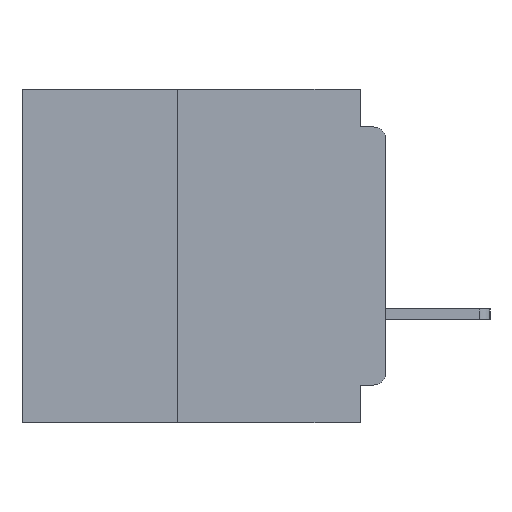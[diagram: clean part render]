
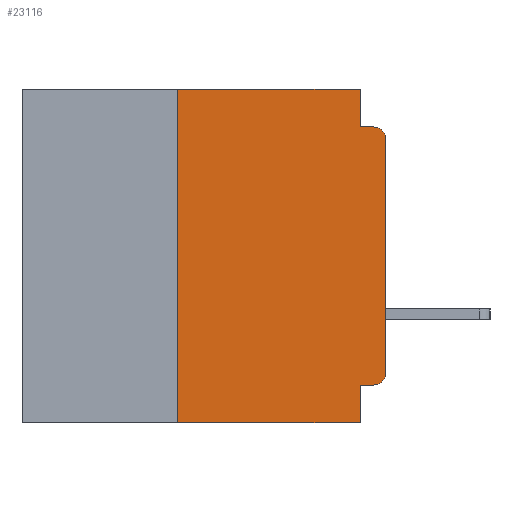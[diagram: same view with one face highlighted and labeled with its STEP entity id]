
A CAD part, left-side view. The second image highlights one B-rep face of the part: STEP entity #23116.
In plain terms, the highlighted planar face has unit normal (-1, 0, 0).
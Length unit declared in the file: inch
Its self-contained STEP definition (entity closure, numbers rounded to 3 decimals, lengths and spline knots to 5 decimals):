
#888 = EDGE_CURVE ( 'NONE', #4619, #17819, #34045, .T. ) ;
#2094 = CIRCLE ( 'NONE', #13594, 0.015 ) ;
#2115 = CARTESIAN_POINT ( 'NONE',  ( 0., 0.031, -0.4 ) ) ;
#2514 = CARTESIAN_POINT ( 'NONE',  ( 0., 0.031, -0.355 ) ) ;
#3103 = EDGE_CURVE ( 'NONE', #8477, #9097, #13351, .T. ) ;
#3969 = LINE ( 'NONE', #42979, #28569 ) ;
#4619 = VERTEX_POINT ( 'NONE', #24319 ) ;
#5118 = CARTESIAN_POINT ( 'NONE',  ( 0., 0.031, 0. ) ) ;
#5341 = DIRECTION ( 'NONE',  ( 0., 0., 1. ) ) ;
#5446 = EDGE_CURVE ( 'NONE', #5993, #7197, #28767, .T. ) ;
#5721 = VECTOR ( 'NONE', #15333, 39.37008 ) ;
#5993 = VERTEX_POINT ( 'NONE', #18700 ) ;
#6261 = CARTESIAN_POINT ( 'NONE',  ( 0., 0.031, -0.045 ) ) ;
#6871 = VECTOR ( 'NONE', #11600, 39.37008 ) ;
#7197 = VERTEX_POINT ( 'NONE', #2514 ) ;
#7807 = AXIS2_PLACEMENT_3D ( 'NONE', #40849, #14601, #37731 ) ;
#7888 = AXIS2_PLACEMENT_3D ( 'NONE', #30933, #22339, #20703 ) ;
#8477 = VERTEX_POINT ( 'NONE', #26603 ) ;
#8787 = ORIENTED_EDGE ( 'NONE', *, *, #8852, .F. ) ;
#8852 = EDGE_CURVE ( 'NONE', #7197, #25153, #23543, .T. ) ;
#8934 = CARTESIAN_POINT ( 'NONE',  ( 0., 0.031, -0.4 ) ) ;
#9097 = VERTEX_POINT ( 'NONE', #16725 ) ;
#10554 = ORIENTED_EDGE ( 'NONE', *, *, #17882, .F. ) ;
#10706 = CARTESIAN_POINT ( 'NONE',  ( 0., 0.015, -0.34 ) ) ;
#11222 = PLANE ( 'NONE',  #7807 ) ;
#11600 = DIRECTION ( 'NONE',  ( 0., -1., 0. ) ) ;
#11652 = EDGE_LOOP ( 'NONE', ( #22100, #34295, #29966, #24642, #14108, #10554, #26506, #8787, #36205, #35474 ) ) ;
#11753 = CARTESIAN_POINT ( 'NONE',  ( 0., 0.015, -0.045 ) ) ;
#12036 = CARTESIAN_POINT ( 'NONE',  ( 0., 0.25, -0.4 ) ) ;
#13015 = VERTEX_POINT ( 'NONE', #6261 ) ;
#13351 = LINE ( 'NONE', #34385, #38707 ) ;
#13594 = AXIS2_PLACEMENT_3D ( 'NONE', #10706, #33955, #14080 ) ;
#14080 = DIRECTION ( 'NONE',  ( 0., 0., -1. ) ) ;
#14108 = ORIENTED_EDGE ( 'NONE', *, *, #3103, .F. ) ;
#14601 = DIRECTION ( 'NONE',  ( 1., 0., 0. ) ) ;
#14740 = LINE ( 'NONE', #5118, #5721 ) ;
#15333 = DIRECTION ( 'NONE',  ( 0., 0., -1. ) ) ;
#15645 = EDGE_CURVE ( 'NONE', #39787, #25153, #3969, .T. ) ;
#15729 = VECTOR ( 'NONE', #28876, 39.37008 ) ;
#16725 = CARTESIAN_POINT ( 'NONE',  ( 0., 0.031, 0. ) ) ;
#17139 = DIRECTION ( 'NONE',  ( 0., 0., 1. ) ) ;
#17592 = FACE_OUTER_BOUND ( 'NONE', #11652, .T. ) ;
#17819 = VERTEX_POINT ( 'NONE', #11753 ) ;
#17882 = EDGE_CURVE ( 'NONE', #39787, #8477, #35673, .T. ) ;
#18700 = CARTESIAN_POINT ( 'NONE',  ( 0., 0.015, -0.355 ) ) ;
#20130 = EDGE_CURVE ( 'NONE', #9097, #13015, #14740, .T. ) ;
#20703 = DIRECTION ( 'NONE',  ( 0., 0., -1. ) ) ;
#22100 = ORIENTED_EDGE ( 'NONE', *, *, #41073, .T. ) ;
#22215 = CARTESIAN_POINT ( 'NONE',  ( 0., 0.25, -0.4 ) ) ;
#22339 = DIRECTION ( 'NONE',  ( -1., 0., 0. ) ) ;
#22647 = DIRECTION ( 'NONE',  ( 0., 1., 0. ) ) ;
#23116 = ADVANCED_FACE ( 'NONE', ( #17592 ), #11222, .F. ) ;
#23303 = DIRECTION ( 'NONE',  ( 0., -1., 0. ) ) ;
#23543 = LINE ( 'NONE', #8934, #15729 ) ;
#24319 = CARTESIAN_POINT ( 'NONE',  ( 0., 0., -0.06 ) ) ;
#24642 = ORIENTED_EDGE ( 'NONE', *, *, #20130, .F. ) ;
#25153 = VERTEX_POINT ( 'NONE', #2115 ) ;
#25642 = EDGE_CURVE ( 'NONE', #13015, #17819, #42145, .T. ) ;
#26506 = ORIENTED_EDGE ( 'NONE', *, *, #15645, .T. ) ;
#26603 = CARTESIAN_POINT ( 'NONE',  ( 0., 0.25, 0. ) ) ;
#26873 = VECTOR ( 'NONE', #5341, 39.37008 ) ;
#27188 = VERTEX_POINT ( 'NONE', #35729 ) ;
#28569 = VECTOR ( 'NONE', #23303, 39.37008 ) ;
#28767 = LINE ( 'NONE', #29280, #36529 ) ;
#28876 = DIRECTION ( 'NONE',  ( 0., 0., -1. ) ) ;
#29280 = CARTESIAN_POINT ( 'NONE',  ( 0., 0., -0.355 ) ) ;
#29966 = ORIENTED_EDGE ( 'NONE', *, *, #25642, .F. ) ;
#30933 = CARTESIAN_POINT ( 'NONE',  ( 0., 0.015, -0.06 ) ) ;
#32585 = LINE ( 'NONE', #36933, #40248 ) ;
#33955 = DIRECTION ( 'NONE',  ( -1., 0., 0. ) ) ;
#34045 = CIRCLE ( 'NONE', #7888, 0.015 ) ;
#34295 = ORIENTED_EDGE ( 'NONE', *, *, #888, .T. ) ;
#34385 = CARTESIAN_POINT ( 'NONE',  ( 0., 0.437, 0. ) ) ;
#35066 = DIRECTION ( 'NONE',  ( 0., -1., 0. ) ) ;
#35356 = EDGE_CURVE ( 'NONE', #5993, #27188, #2094, .T. ) ;
#35474 = ORIENTED_EDGE ( 'NONE', *, *, #35356, .T. ) ;
#35673 = LINE ( 'NONE', #12036, #26873 ) ;
#35729 = CARTESIAN_POINT ( 'NONE',  ( 0., 0., -0.34 ) ) ;
#36205 = ORIENTED_EDGE ( 'NONE', *, *, #5446, .F. ) ;
#36529 = VECTOR ( 'NONE', #22647, 39.37008 ) ;
#36933 = CARTESIAN_POINT ( 'NONE',  ( 0., 0., 0. ) ) ;
#37731 = DIRECTION ( 'NONE',  ( 0., 0., -1. ) ) ;
#38707 = VECTOR ( 'NONE', #35066, 39.37008 ) ;
#39787 = VERTEX_POINT ( 'NONE', #22215 ) ;
#40248 = VECTOR ( 'NONE', #17139, 39.37008 ) ;
#40849 = CARTESIAN_POINT ( 'NONE',  ( 0., 0.437, 0. ) ) ;
#41073 = EDGE_CURVE ( 'NONE', #27188, #4619, #32585, .T. ) ;
#41212 = CARTESIAN_POINT ( 'NONE',  ( 0., 0., -0.045 ) ) ;
#42145 = LINE ( 'NONE', #41212, #6871 ) ;
#42979 = CARTESIAN_POINT ( 'NONE',  ( 0., 0.437, -0.4 ) ) ;
